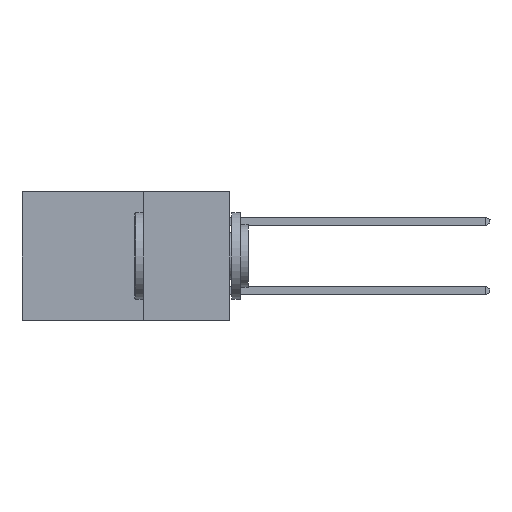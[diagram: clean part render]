
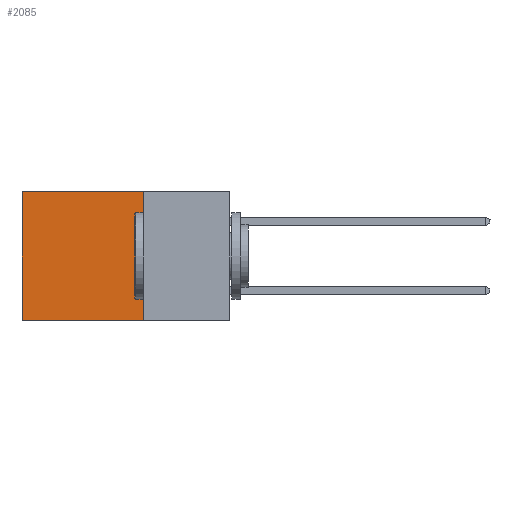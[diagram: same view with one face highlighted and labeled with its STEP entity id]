
A CAD part, left-side view. The second image highlights one B-rep face of the part: STEP entity #2085.
In plain terms, the highlighted planar face has unit normal (-1, 0, 0).
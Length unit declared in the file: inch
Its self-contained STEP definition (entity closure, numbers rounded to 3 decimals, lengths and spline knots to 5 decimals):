
#12 = EDGE_CURVE ( 'NONE', #7307, #463, #1952, .T. ) ;
#124 = EDGE_CURVE ( 'NONE', #1486, #2774, #508, .T. ) ;
#463 = VERTEX_POINT ( 'NONE', #9244 ) ;
#508 = LINE ( 'NONE', #8466, #2999 ) ;
#550 = PLANE ( 'NONE',  #4353 ) ;
#1486 = VERTEX_POINT ( 'NONE', #7192 ) ;
#1668 = ORIENTED_EDGE ( 'NONE', *, *, #6341, .F. ) ;
#1751 = DIRECTION ( 'NONE',  ( 0., 1., 0. ) ) ;
#1818 = ORIENTED_EDGE ( 'NONE', *, *, #12, .T. ) ;
#1952 = LINE ( 'NONE', #4285, #6636 ) ;
#2085 = ADVANCED_FACE ( 'NONE', ( #6759 ), #550, .F. ) ;
#2774 = VERTEX_POINT ( 'NONE', #9697 ) ;
#2999 = VECTOR ( 'NONE', #9158, 39.37008 ) ;
#3470 = LINE ( 'NONE', #8247, #4604 ) ;
#4285 = CARTESIAN_POINT ( 'NONE',  ( 0.2615, 0.25, 0. ) ) ;
#4353 = AXIS2_PLACEMENT_3D ( 'NONE', #6032, #9201, #9042 ) ;
#4604 = VECTOR ( 'NONE', #5147, 39.37008 ) ;
#4809 = EDGE_LOOP ( 'NONE', ( #9659, #6514, #1668, #1818 ) ) ;
#5043 = CARTESIAN_POINT ( 'NONE',  ( 0.2615, 0.25, -0.37 ) ) ;
#5147 = DIRECTION ( 'NONE',  ( 0., 0., -1. ) ) ;
#6032 = CARTESIAN_POINT ( 'NONE',  ( 0.2615, 0.25, -0.37 ) ) ;
#6341 = EDGE_CURVE ( 'NONE', #7307, #1486, #6637, .T. ) ;
#6514 = ORIENTED_EDGE ( 'NONE', *, *, #124, .F. ) ;
#6636 = VECTOR ( 'NONE', #1751, 39.37008 ) ;
#6637 = LINE ( 'NONE', #5043, #7372 ) ;
#6759 = FACE_OUTER_BOUND ( 'NONE', #4809, .T. ) ;
#7192 = CARTESIAN_POINT ( 'NONE',  ( 0.2615, 0.25, -0.37 ) ) ;
#7307 = VERTEX_POINT ( 'NONE', #7598 ) ;
#7372 = VECTOR ( 'NONE', #9125, 39.37008 ) ;
#7598 = CARTESIAN_POINT ( 'NONE',  ( 0.2615, 0.25, 0. ) ) ;
#7865 = EDGE_CURVE ( 'NONE', #463, #2774, #3470, .T. ) ;
#8247 = CARTESIAN_POINT ( 'NONE',  ( 0.2615, 0.6, -0.37 ) ) ;
#8466 = CARTESIAN_POINT ( 'NONE',  ( 0.2615, 0.25, -0.37 ) ) ;
#9042 = DIRECTION ( 'NONE',  ( 0., 0., -1. ) ) ;
#9125 = DIRECTION ( 'NONE',  ( 0., 0., -1. ) ) ;
#9158 = DIRECTION ( 'NONE',  ( 0., 1., 0. ) ) ;
#9201 = DIRECTION ( 'NONE',  ( 1., 0., 0. ) ) ;
#9244 = CARTESIAN_POINT ( 'NONE',  ( 0.2615, 0.6, 0. ) ) ;
#9659 = ORIENTED_EDGE ( 'NONE', *, *, #7865, .T. ) ;
#9697 = CARTESIAN_POINT ( 'NONE',  ( 0.2615, 0.6, -0.37 ) ) ;
